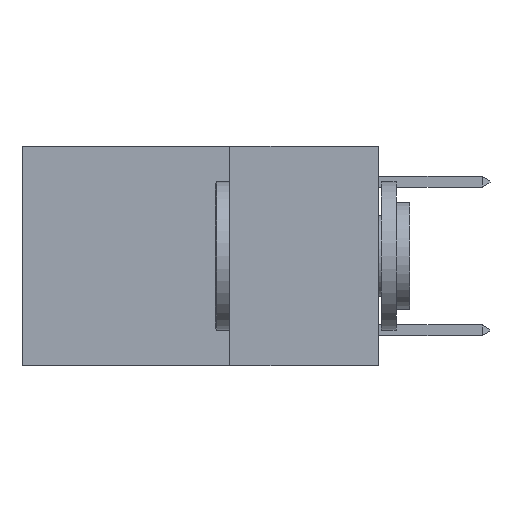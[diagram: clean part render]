
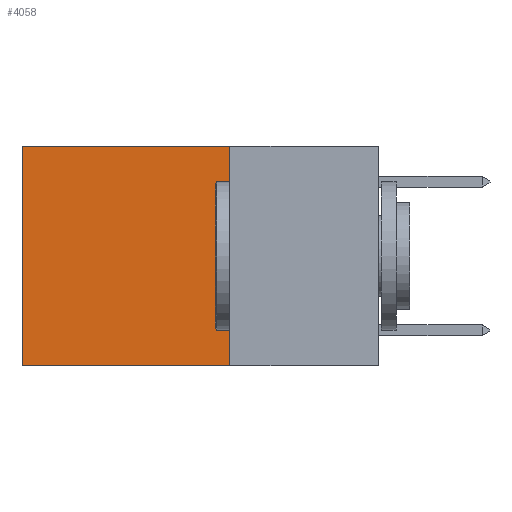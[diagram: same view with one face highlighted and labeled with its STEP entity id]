
A CAD part, left-side view. The second image highlights one B-rep face of the part: STEP entity #4058.
In plain terms, the highlighted planar face has unit normal (-1, 0, 0).
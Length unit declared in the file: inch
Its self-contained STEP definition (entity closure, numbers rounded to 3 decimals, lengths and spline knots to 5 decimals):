
#267 = VERTEX_POINT ( 'NONE', #11125 ) ;
#1080 = DIRECTION ( 'NONE',  ( 0., 0., -1. ) ) ;
#1310 = VECTOR ( 'NONE', #5765, 39.37008 ) ;
#2013 = VECTOR ( 'NONE', #10042, 39.37008 ) ;
#2630 = CARTESIAN_POINT ( 'NONE',  ( 0.2625, 0.25, 0. ) ) ;
#3293 = VERTEX_POINT ( 'NONE', #9319 ) ;
#3498 = LINE ( 'NONE', #2630, #5904 ) ;
#3885 = CARTESIAN_POINT ( 'NONE',  ( 0.2625, 0.25, -0.37 ) ) ;
#4058 = ADVANCED_FACE ( 'NONE', ( #6580 ), #11241, .F. ) ;
#5004 = LINE ( 'NONE', #3885, #2013 ) ;
#5346 = DIRECTION ( 'NONE',  ( 0., 1., 0. ) ) ;
#5683 = DIRECTION ( 'NONE',  ( 0., 0., -1. ) ) ;
#5765 = DIRECTION ( 'NONE',  ( 0., 0., -1. ) ) ;
#5904 = VECTOR ( 'NONE', #5683, 39.37008 ) ;
#5929 = ORIENTED_EDGE ( 'NONE', *, *, #10358, .F. ) ;
#6227 = ORIENTED_EDGE ( 'NONE', *, *, #8090, .T. ) ;
#6252 = EDGE_CURVE ( 'NONE', #6771, #9770, #6707, .T. ) ;
#6580 = FACE_OUTER_BOUND ( 'NONE', #13163, .T. ) ;
#6707 = LINE ( 'NONE', #7865, #1310 ) ;
#6771 = VERTEX_POINT ( 'NONE', #10264 ) ;
#7134 = CARTESIAN_POINT ( 'NONE',  ( 0.2625, 0.25, 0. ) ) ;
#7160 = VECTOR ( 'NONE', #5346, 39.37008 ) ;
#7182 = DIRECTION ( 'NONE',  ( 1., 0., 0. ) ) ;
#7461 = LINE ( 'NONE', #9518, #7160 ) ;
#7865 = CARTESIAN_POINT ( 'NONE',  ( 0.2625, 0.6, 0. ) ) ;
#8090 = EDGE_CURVE ( 'NONE', #267, #6771, #7461, .T. ) ;
#8716 = ORIENTED_EDGE ( 'NONE', *, *, #13102, .F. ) ;
#9272 = AXIS2_PLACEMENT_3D ( 'NONE', #7134, #7182, #1080 ) ;
#9319 = CARTESIAN_POINT ( 'NONE',  ( 0.2625, 0.25, -0.37 ) ) ;
#9518 = CARTESIAN_POINT ( 'NONE',  ( 0.2625, 0.25, 0. ) ) ;
#9770 = VERTEX_POINT ( 'NONE', #11238 ) ;
#10042 = DIRECTION ( 'NONE',  ( 0., 1., 0. ) ) ;
#10264 = CARTESIAN_POINT ( 'NONE',  ( 0.2625, 0.6, 0. ) ) ;
#10358 = EDGE_CURVE ( 'NONE', #3293, #9770, #5004, .T. ) ;
#11057 = ORIENTED_EDGE ( 'NONE', *, *, #6252, .T. ) ;
#11125 = CARTESIAN_POINT ( 'NONE',  ( 0.2625, 0.25, 0. ) ) ;
#11238 = CARTESIAN_POINT ( 'NONE',  ( 0.2625, 0.6, -0.37 ) ) ;
#11241 = PLANE ( 'NONE',  #9272 ) ;
#13102 = EDGE_CURVE ( 'NONE', #267, #3293, #3498, .T. ) ;
#13163 = EDGE_LOOP ( 'NONE', ( #11057, #5929, #8716, #6227 ) ) ;
